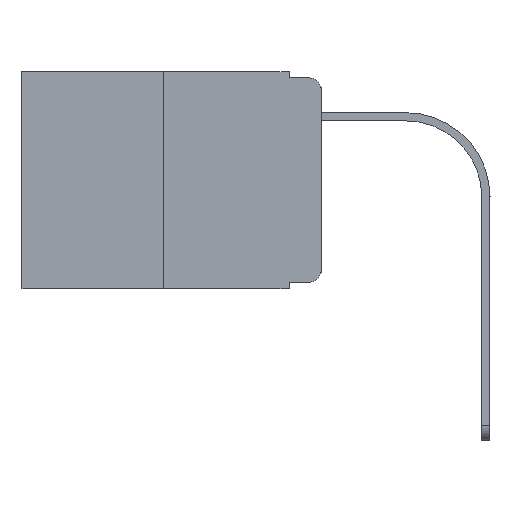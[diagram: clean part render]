
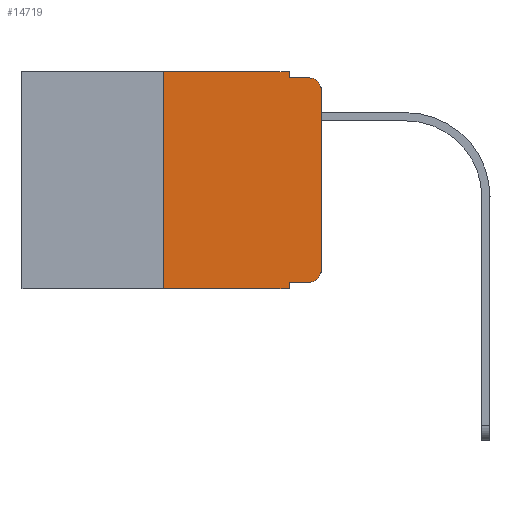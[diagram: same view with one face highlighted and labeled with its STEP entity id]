
A CAD part, left-side view. The second image highlights one B-rep face of the part: STEP entity #14719.
In plain terms, the highlighted planar face has unit normal (-1, 0, 0).
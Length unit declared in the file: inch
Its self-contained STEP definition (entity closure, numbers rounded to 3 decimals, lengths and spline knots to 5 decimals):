
#462 = LINE ( 'NONE', #2292, #6062 ) ;
#966 = CARTESIAN_POINT ( 'NONE',  ( 0., 0.473, 0. ) ) ;
#1044 = CARTESIAN_POINT ( 'NONE',  ( 0., 0., 0. ) ) ;
#1234 = CARTESIAN_POINT ( 'NONE',  ( 0., 0.25, 0. ) ) ;
#1547 = CARTESIAN_POINT ( 'NONE',  ( 0., 0.051, -0.01 ) ) ;
#1682 = CARTESIAN_POINT ( 'NONE',  ( 0., 0.473, 0. ) ) ;
#2081 = ORIENTED_EDGE ( 'NONE', *, *, #10082, .F. ) ;
#2085 = DIRECTION ( 'NONE',  ( 0., 0., -1. ) ) ;
#2292 = CARTESIAN_POINT ( 'NONE',  ( 0., 0.051, 0. ) ) ;
#2579 = AXIS2_PLACEMENT_3D ( 'NONE', #12230, #4917, #2085 ) ;
#2591 = ORIENTED_EDGE ( 'NONE', *, *, #11587, .T. ) ;
#2632 = CARTESIAN_POINT ( 'NONE',  ( 0., 0., -0.313 ) ) ;
#2850 = VERTEX_POINT ( 'NONE', #12116 ) ;
#2992 = DIRECTION ( 'NONE',  ( 0., 0., -1. ) ) ;
#3441 = DIRECTION ( 'NONE',  ( 0., 0., -1. ) ) ;
#3526 = DIRECTION ( 'NONE',  ( 0., -1., 0. ) ) ;
#3549 = ORIENTED_EDGE ( 'NONE', *, *, #18448, .F. ) ;
#3584 = VECTOR ( 'NONE', #15155, 39.37008 ) ;
#3790 = EDGE_CURVE ( 'NONE', #2850, #11617, #462, .T. ) ;
#3819 = VECTOR ( 'NONE', #2992, 39.37008 ) ;
#3922 = DIRECTION ( 'NONE',  ( 0., 0., -1. ) ) ;
#4274 = VERTEX_POINT ( 'NONE', #5480 ) ;
#4487 = CARTESIAN_POINT ( 'NONE',  ( 0., 0.051, -0.333 ) ) ;
#4759 = CARTESIAN_POINT ( 'NONE',  ( 0., 0.25, -0.343 ) ) ;
#4784 = VECTOR ( 'NONE', #17850, 39.37008 ) ;
#4917 = DIRECTION ( 'NONE',  ( -1., 0., 0. ) ) ;
#4928 = VERTEX_POINT ( 'NONE', #4759 ) ;
#5480 = CARTESIAN_POINT ( 'NONE',  ( 0., 0.051, 0. ) ) ;
#5778 = VERTEX_POINT ( 'NONE', #11507 ) ;
#5814 = LINE ( 'NONE', #4487, #10024 ) ;
#6062 = VECTOR ( 'NONE', #3441, 39.37008 ) ;
#6141 = VERTEX_POINT ( 'NONE', #2632 ) ;
#6219 = EDGE_CURVE ( 'NONE', #10741, #5778, #17796, .T. ) ;
#6795 = ORIENTED_EDGE ( 'NONE', *, *, #10471, .F. ) ;
#7080 = CARTESIAN_POINT ( 'NONE',  ( 0., 0.02, -0.03 ) ) ;
#7583 = VECTOR ( 'NONE', #18544, 39.37008 ) ;
#7791 = ORIENTED_EDGE ( 'NONE', *, *, #11212, .T. ) ;
#8303 = ORIENTED_EDGE ( 'NONE', *, *, #17896, .T. ) ;
#8343 = VECTOR ( 'NONE', #3526, 39.37008 ) ;
#8542 = DIRECTION ( 'NONE',  ( 0., 0., -1. ) ) ;
#9027 = LINE ( 'NONE', #1682, #4784 ) ;
#9170 = LINE ( 'NONE', #10892, #8343 ) ;
#9182 = LINE ( 'NONE', #11879, #3819 ) ;
#9366 = ORIENTED_EDGE ( 'NONE', *, *, #14894, .F. ) ;
#10024 = VECTOR ( 'NONE', #17514, 39.37008 ) ;
#10065 = VERTEX_POINT ( 'NONE', #1234 ) ;
#10082 = EDGE_CURVE ( 'NONE', #4928, #10065, #14608, .T. ) ;
#10471 = EDGE_CURVE ( 'NONE', #10065, #4274, #9027, .T. ) ;
#10623 = EDGE_CURVE ( 'NONE', #4928, #11617, #13620, .T. ) ;
#10741 = VERTEX_POINT ( 'NONE', #11323 ) ;
#10817 = CIRCLE ( 'NONE', #2579, 0.02 ) ;
#10892 = CARTESIAN_POINT ( 'NONE',  ( 0., 0.051, -0.01 ) ) ;
#11212 = EDGE_CURVE ( 'NONE', #2850, #17088, #5814, .T. ) ;
#11261 = VERTEX_POINT ( 'NONE', #1547 ) ;
#11323 = CARTESIAN_POINT ( 'NONE',  ( 0., 0., -0.03 ) ) ;
#11382 = FACE_OUTER_BOUND ( 'NONE', #14664, .T. ) ;
#11507 = CARTESIAN_POINT ( 'NONE',  ( 0., 0.02, -0.01 ) ) ;
#11587 = EDGE_CURVE ( 'NONE', #6141, #10741, #14136, .T. ) ;
#11617 = VERTEX_POINT ( 'NONE', #15393 ) ;
#11640 = DIRECTION ( 'NONE',  ( 0., 0., 1. ) ) ;
#11792 = DIRECTION ( 'NONE',  ( -1., 0., 0. ) ) ;
#11879 = CARTESIAN_POINT ( 'NONE',  ( 0., 0.051, 0. ) ) ;
#12116 = CARTESIAN_POINT ( 'NONE',  ( 0., 0.051, -0.333 ) ) ;
#12230 = CARTESIAN_POINT ( 'NONE',  ( 0., 0.02, -0.313 ) ) ;
#12540 = DIRECTION ( 'NONE',  ( 1., 0., 0. ) ) ;
#12858 = ORIENTED_EDGE ( 'NONE', *, *, #3790, .F. ) ;
#13620 = LINE ( 'NONE', #13723, #3584 ) ;
#13650 = VECTOR ( 'NONE', #11640, 39.37008 ) ;
#13723 = CARTESIAN_POINT ( 'NONE',  ( 0., 0.473, -0.343 ) ) ;
#13842 = ORIENTED_EDGE ( 'NONE', *, *, #6219, .T. ) ;
#14136 = LINE ( 'NONE', #1044, #7583 ) ;
#14608 = LINE ( 'NONE', #14698, #13650 ) ;
#14664 = EDGE_LOOP ( 'NONE', ( #2591, #13842, #9366, #3549, #6795, #2081, #17379, #12858, #7791, #8303 ) ) ;
#14698 = CARTESIAN_POINT ( 'NONE',  ( 0., 0.25, 0. ) ) ;
#14719 = ADVANCED_FACE ( 'NONE', ( #11382 ), #16852, .F. ) ;
#14871 = CARTESIAN_POINT ( 'NONE',  ( 0., 0.02, -0.333 ) ) ;
#14894 = EDGE_CURVE ( 'NONE', #11261, #5778, #9170, .T. ) ;
#15155 = DIRECTION ( 'NONE',  ( 0., -1., 0. ) ) ;
#15393 = CARTESIAN_POINT ( 'NONE',  ( 0., 0.051, -0.343 ) ) ;
#16852 = PLANE ( 'NONE',  #17505 ) ;
#16875 = AXIS2_PLACEMENT_3D ( 'NONE', #7080, #11792, #8542 ) ;
#17088 = VERTEX_POINT ( 'NONE', #14871 ) ;
#17379 = ORIENTED_EDGE ( 'NONE', *, *, #10623, .T. ) ;
#17505 = AXIS2_PLACEMENT_3D ( 'NONE', #966, #12540, #3922 ) ;
#17514 = DIRECTION ( 'NONE',  ( 0., -1., 0. ) ) ;
#17796 = CIRCLE ( 'NONE', #16875, 0.02 ) ;
#17850 = DIRECTION ( 'NONE',  ( 0., -1., 0. ) ) ;
#17896 = EDGE_CURVE ( 'NONE', #17088, #6141, #10817, .T. ) ;
#18448 = EDGE_CURVE ( 'NONE', #4274, #11261, #9182, .T. ) ;
#18544 = DIRECTION ( 'NONE',  ( 0., 0., 1. ) ) ;
